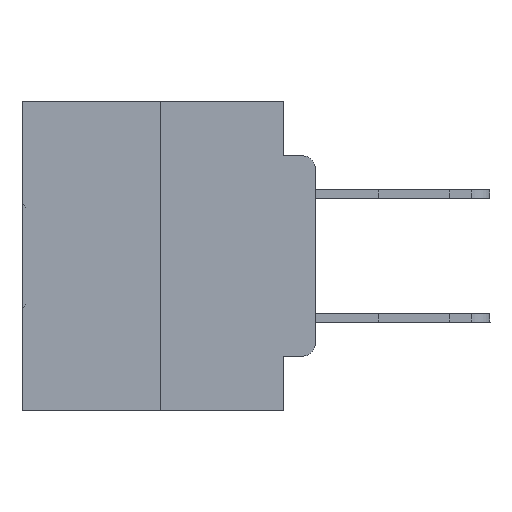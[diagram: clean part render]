
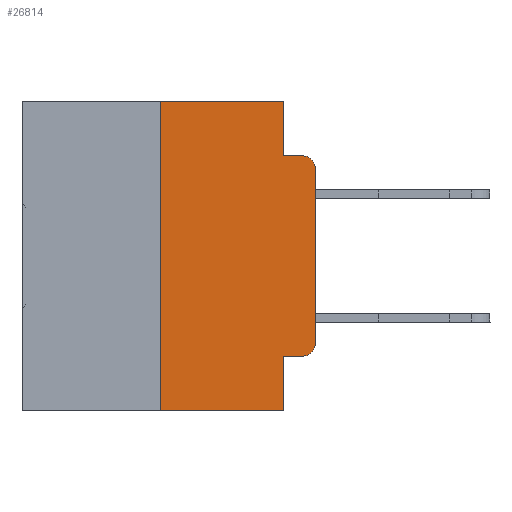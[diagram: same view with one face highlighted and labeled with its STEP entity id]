
A CAD part, left-side view. The second image highlights one B-rep face of the part: STEP entity #26814.
In plain terms, the highlighted planar face has unit normal (-1, 0, 0).
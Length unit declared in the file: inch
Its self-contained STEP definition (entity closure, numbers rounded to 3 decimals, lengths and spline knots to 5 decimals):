
#13 = EDGE_CURVE ( 'NONE', #30282, #1297, #4645, .T. ) ;
#58 = LINE ( 'NONE', #26441, #13872 ) ;
#728 = CARTESIAN_POINT ( 'NONE',  ( 0., 0.02, -0.1085 ) ) ;
#1226 = DIRECTION ( 'NONE',  ( 0., 0., 1. ) ) ;
#1297 = VERTEX_POINT ( 'NONE', #23644 ) ;
#1373 = ORIENTED_EDGE ( 'NONE', *, *, #10809, .F. ) ;
#1472 = CIRCLE ( 'NONE', #25041, 0.02 ) ;
#1491 = CARTESIAN_POINT ( 'NONE',  ( 0., 0.473, 0. ) ) ;
#2310 = PLANE ( 'NONE',  #29509 ) ;
#3502 = CARTESIAN_POINT ( 'NONE',  ( 0., 0., -0.1085 ) ) ;
#3518 = EDGE_CURVE ( 'NONE', #29785, #11080, #6335, .T. ) ;
#3993 = ORIENTED_EDGE ( 'NONE', *, *, #32515, .T. ) ;
#4642 = DIRECTION ( 'NONE',  ( 1., 0., 0. ) ) ;
#4645 = LINE ( 'NONE', #1491, #29173 ) ;
#4793 = CIRCLE ( 'NONE', #31107, 0.02 ) ;
#5626 = DIRECTION ( 'NONE',  ( 0., -1., 0. ) ) ;
#6112 = VECTOR ( 'NONE', #5626, 39.37008 ) ;
#6335 = LINE ( 'NONE', #16681, #11477 ) ;
#6337 = DIRECTION ( 'NONE',  ( 0., -1., 0. ) ) ;
#7002 = VERTEX_POINT ( 'NONE', #28881 ) ;
#7165 = ORIENTED_EDGE ( 'NONE', *, *, #13, .F. ) ;
#7350 = CARTESIAN_POINT ( 'NONE',  ( 0., 0.25, 0. ) ) ;
#7396 = DIRECTION ( 'NONE',  ( 0., 0., -1. ) ) ;
#7422 = CARTESIAN_POINT ( 'NONE',  ( 0., 0.02, -0.3915 ) ) ;
#7719 = DIRECTION ( 'NONE',  ( 0., -1., 0. ) ) ;
#7838 = LINE ( 'NONE', #7350, #23271 ) ;
#7950 = LINE ( 'NONE', #17558, #21821 ) ;
#8712 = DIRECTION ( 'NONE',  ( 0., 0., -1. ) ) ;
#9486 = ORIENTED_EDGE ( 'NONE', *, *, #3518, .T. ) ;
#9626 = EDGE_CURVE ( 'NONE', #7002, #17179, #28324, .T. ) ;
#10688 = CARTESIAN_POINT ( 'NONE',  ( 0., 0.25, -0.5 ) ) ;
#10809 = EDGE_CURVE ( 'NONE', #32682, #17442, #30583, .T. ) ;
#11080 = VERTEX_POINT ( 'NONE', #3502 ) ;
#11477 = VECTOR ( 'NONE', #16909, 39.37008 ) ;
#11663 = CARTESIAN_POINT ( 'NONE',  ( 0., 0.02, -0.4115 ) ) ;
#12176 = EDGE_CURVE ( 'NONE', #14729, #30282, #7838, .T. ) ;
#13736 = VERTEX_POINT ( 'NONE', #11663 ) ;
#13872 = VECTOR ( 'NONE', #8712, 39.37008 ) ;
#14729 = VERTEX_POINT ( 'NONE', #10688 ) ;
#15631 = DIRECTION ( 'NONE',  ( 0., 0., -1. ) ) ;
#16023 = CARTESIAN_POINT ( 'NONE',  ( 0., 0.051, -0.0885 ) ) ;
#16519 = EDGE_CURVE ( 'NONE', #13736, #29785, #4793, .T. ) ;
#16681 = CARTESIAN_POINT ( 'NONE',  ( 0., 0., 0. ) ) ;
#16909 = DIRECTION ( 'NONE',  ( 0., 0., 1. ) ) ;
#17179 = VERTEX_POINT ( 'NONE', #28184 ) ;
#17368 = DIRECTION ( 'NONE',  ( -1., 0., 0. ) ) ;
#17442 = VERTEX_POINT ( 'NONE', #21545 ) ;
#17558 = CARTESIAN_POINT ( 'NONE',  ( 0., 0.473, -0.5 ) ) ;
#17993 = VECTOR ( 'NONE', #26496, 39.37008 ) ;
#18729 = ORIENTED_EDGE ( 'NONE', *, *, #9626, .F. ) ;
#19155 = ORIENTED_EDGE ( 'NONE', *, *, #25272, .T. ) ;
#21545 = CARTESIAN_POINT ( 'NONE',  ( 0., 0.02, -0.0885 ) ) ;
#21821 = VECTOR ( 'NONE', #7719, 39.37008 ) ;
#22904 = EDGE_CURVE ( 'NONE', #1297, #32682, #58, .T. ) ;
#23271 = VECTOR ( 'NONE', #1226, 39.37008 ) ;
#23407 = CARTESIAN_POINT ( 'NONE',  ( 0., 0.051, -0.0885 ) ) ;
#23440 = CARTESIAN_POINT ( 'NONE',  ( 0., 0.051, -0.4115 ) ) ;
#23644 = CARTESIAN_POINT ( 'NONE',  ( 0., 0.051, 0. ) ) ;
#25041 = AXIS2_PLACEMENT_3D ( 'NONE', #728, #31139, #15631 ) ;
#25272 = EDGE_CURVE ( 'NONE', #11080, #17442, #1472, .T. ) ;
#25357 = ORIENTED_EDGE ( 'NONE', *, *, #22904, .F. ) ;
#25445 = ORIENTED_EDGE ( 'NONE', *, *, #12176, .F. ) ;
#25470 = ORIENTED_EDGE ( 'NONE', *, *, #16519, .T. ) ;
#26364 = EDGE_CURVE ( 'NONE', #7002, #13736, #31442, .T. ) ;
#26441 = CARTESIAN_POINT ( 'NONE',  ( 0., 0.051, 0. ) ) ;
#26496 = DIRECTION ( 'NONE',  ( 0., 0., -1. ) ) ;
#26814 = ADVANCED_FACE ( 'NONE', ( #32602 ), #2310, .F. ) ;
#26850 = EDGE_LOOP ( 'NONE', ( #9486, #19155, #1373, #25357, #7165, #25445, #3993, #18729, #28069, #25470 ) ) ;
#27459 = DIRECTION ( 'NONE',  ( 0., 0., -1. ) ) ;
#27971 = CARTESIAN_POINT ( 'NONE',  ( 0., 0., -0.3915 ) ) ;
#28069 = ORIENTED_EDGE ( 'NONE', *, *, #26364, .T. ) ;
#28184 = CARTESIAN_POINT ( 'NONE',  ( 0., 0.051, -0.5 ) ) ;
#28324 = LINE ( 'NONE', #28920, #17993 ) ;
#28881 = CARTESIAN_POINT ( 'NONE',  ( 0., 0.051, -0.4115 ) ) ;
#28920 = CARTESIAN_POINT ( 'NONE',  ( 0., 0.051, 0. ) ) ;
#29013 = VECTOR ( 'NONE', #29458, 39.37008 ) ;
#29173 = VECTOR ( 'NONE', #6337, 39.37008 ) ;
#29458 = DIRECTION ( 'NONE',  ( 0., -1., 0. ) ) ;
#29509 = AXIS2_PLACEMENT_3D ( 'NONE', #32365, #4642, #7396 ) ;
#29785 = VERTEX_POINT ( 'NONE', #27971 ) ;
#30282 = VERTEX_POINT ( 'NONE', #32216 ) ;
#30583 = LINE ( 'NONE', #16023, #29013 ) ;
#31107 = AXIS2_PLACEMENT_3D ( 'NONE', #7422, #17368, #27459 ) ;
#31139 = DIRECTION ( 'NONE',  ( -1., 0., 0. ) ) ;
#31442 = LINE ( 'NONE', #23440, #6112 ) ;
#32216 = CARTESIAN_POINT ( 'NONE',  ( 0., 0.25, 0. ) ) ;
#32365 = CARTESIAN_POINT ( 'NONE',  ( 0., 0.473, 0. ) ) ;
#32515 = EDGE_CURVE ( 'NONE', #14729, #17179, #7950, .T. ) ;
#32602 = FACE_OUTER_BOUND ( 'NONE', #26850, .T. ) ;
#32682 = VERTEX_POINT ( 'NONE', #23407 ) ;
